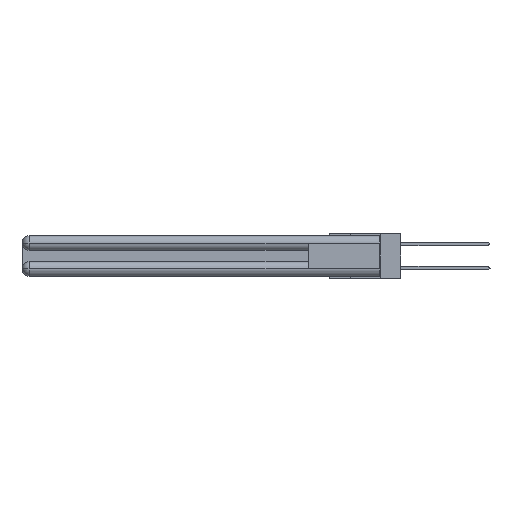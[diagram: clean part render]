
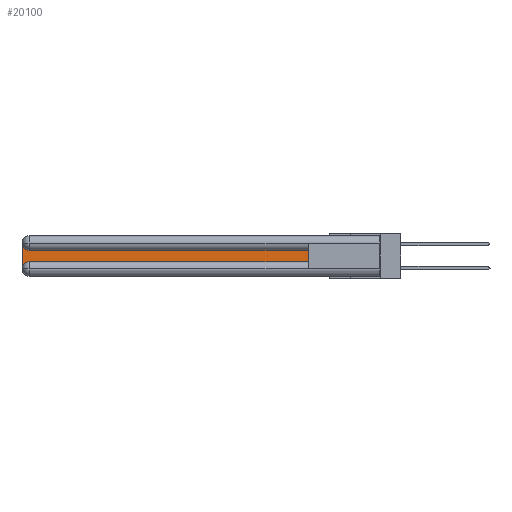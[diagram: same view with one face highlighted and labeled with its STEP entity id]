
A CAD part, left-side view. The second image highlights one B-rep face of the part: STEP entity #20100.
In plain terms, the highlighted planar face has unit normal (-1, 0, 0).
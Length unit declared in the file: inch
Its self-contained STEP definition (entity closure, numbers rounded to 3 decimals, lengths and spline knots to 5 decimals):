
#880 = AXIS2_PLACEMENT_3D ( 'NONE', #8221, #26503, #10858 ) ;
#984 = ORIENTED_EDGE ( 'NONE', *, *, #33386, .T. ) ;
#2043 = VERTEX_POINT ( 'NONE', #3407 ) ;
#2135 = CARTESIAN_POINT ( 'NONE',  ( 0.075, 3., -0.2775 ) ) ;
#2678 = DIRECTION ( 'NONE',  ( 1., 0., 0. ) ) ;
#3407 = CARTESIAN_POINT ( 'NONE',  ( 0.075, 0.6, -0.2175 ) ) ;
#3671 = DIRECTION ( 'NONE',  ( 0., 0., -1. ) ) ;
#4863 = DIRECTION ( 'NONE',  ( 0., 0., -1. ) ) ;
#5138 = VECTOR ( 'NONE', #6829, 39.37008 ) ;
#5446 = DIRECTION ( 'NONE',  ( 0., 0., -1. ) ) ;
#5536 = LINE ( 'NONE', #31433, #8016 ) ;
#5653 = VECTOR ( 'NONE', #21169, 39.37008 ) ;
#5789 = EDGE_LOOP ( 'NONE', ( #984, #30618, #14780, #20889, #17982, #9978 ) ) ;
#5811 = EDGE_CURVE ( 'NONE', #7644, #19074, #12342, .T. ) ;
#5879 = VERTEX_POINT ( 'NONE', #12495 ) ;
#6386 = CARTESIAN_POINT ( 'NONE',  ( 0.075, 0.6, -0.2175 ) ) ;
#6540 = CARTESIAN_POINT ( 'NONE',  ( 0.075, 2.94, -0.0625 ) ) ;
#6829 = DIRECTION ( 'NONE',  ( 0., 0., 1. ) ) ;
#7480 = EDGE_CURVE ( 'NONE', #14312, #21794, #28567, .T. ) ;
#7632 = DIRECTION ( 'NONE',  ( 0., 1., 0. ) ) ;
#7644 = VERTEX_POINT ( 'NONE', #13457 ) ;
#8016 = VECTOR ( 'NONE', #5446, 39.37008 ) ;
#8221 = CARTESIAN_POINT ( 'NONE',  ( 0.075, 3., -0.1225 ) ) ;
#8446 = LINE ( 'NONE', #6386, #5138 ) ;
#8939 = AXIS2_PLACEMENT_3D ( 'NONE', #15762, #2678, #4863 ) ;
#9978 = ORIENTED_EDGE ( 'NONE', *, *, #26239, .T. ) ;
#10858 = DIRECTION ( 'NONE',  ( 0., 0., -1. ) ) ;
#11628 = FACE_OUTER_BOUND ( 'NONE', #5789, .T. ) ;
#12342 = CIRCLE ( 'NONE', #21545, 0.06 ) ;
#12441 = CARTESIAN_POINT ( 'NONE',  ( 0.075, 0.6, -0.1225 ) ) ;
#12495 = CARTESIAN_POINT ( 'NONE',  ( 0.075, 0.6, -0.1225 ) ) ;
#13457 = CARTESIAN_POINT ( 'NONE',  ( 0.075, 2.94, -0.1225 ) ) ;
#13460 = LINE ( 'NONE', #25940, #5653 ) ;
#14312 = VERTEX_POINT ( 'NONE', #2135 ) ;
#14467 = EDGE_CURVE ( 'NONE', #21794, #2043, #13460, .T. ) ;
#14780 = ORIENTED_EDGE ( 'NONE', *, *, #26577, .T. ) ;
#14913 = CARTESIAN_POINT ( 'NONE',  ( 0.075, 3., -0.0625 ) ) ;
#15762 = CARTESIAN_POINT ( 'NONE',  ( 0.075, 2.94, -0.2775 ) ) ;
#17982 = ORIENTED_EDGE ( 'NONE', *, *, #14467, .T. ) ;
#19074 = VERTEX_POINT ( 'NONE', #14913 ) ;
#19243 = DIRECTION ( 'NONE',  ( 1., 0., 0. ) ) ;
#20100 = ADVANCED_FACE ( 'NONE', ( #11628 ), #23903, .F. ) ;
#20889 = ORIENTED_EDGE ( 'NONE', *, *, #7480, .T. ) ;
#21169 = DIRECTION ( 'NONE',  ( 0., -1., 0. ) ) ;
#21545 = AXIS2_PLACEMENT_3D ( 'NONE', #6540, #19243, #3671 ) ;
#21794 = VERTEX_POINT ( 'NONE', #31963 ) ;
#23903 = PLANE ( 'NONE',  #880 ) ;
#24791 = LINE ( 'NONE', #12441, #33353 ) ;
#25940 = CARTESIAN_POINT ( 'NONE',  ( 0.075, 0.6, -0.2175 ) ) ;
#26239 = EDGE_CURVE ( 'NONE', #2043, #5879, #8446, .T. ) ;
#26503 = DIRECTION ( 'NONE',  ( 1., 0., 0. ) ) ;
#26577 = EDGE_CURVE ( 'NONE', #19074, #14312, #5536, .T. ) ;
#28567 = CIRCLE ( 'NONE', #8939, 0.06 ) ;
#30618 = ORIENTED_EDGE ( 'NONE', *, *, #5811, .T. ) ;
#31433 = CARTESIAN_POINT ( 'NONE',  ( 0.075, 3., -0.2175 ) ) ;
#31963 = CARTESIAN_POINT ( 'NONE',  ( 0.075, 2.94, -0.2175 ) ) ;
#33353 = VECTOR ( 'NONE', #7632, 39.37008 ) ;
#33386 = EDGE_CURVE ( 'NONE', #5879, #7644, #24791, .T. ) ;
